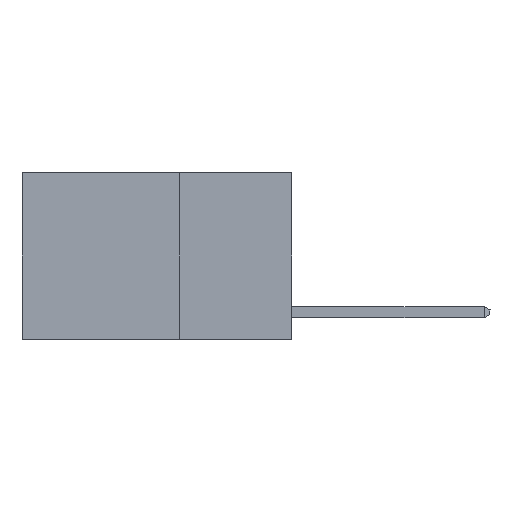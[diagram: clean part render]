
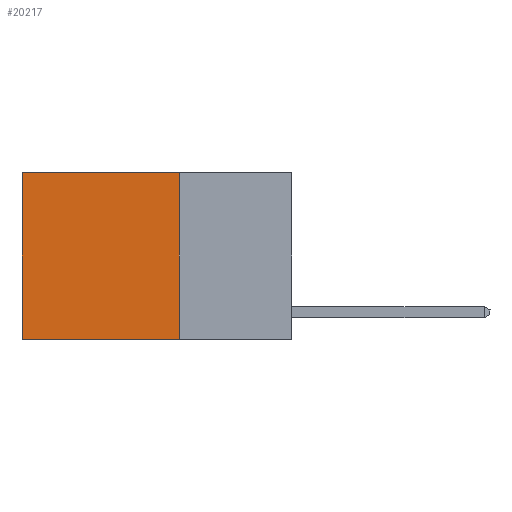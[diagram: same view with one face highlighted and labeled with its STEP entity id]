
A CAD part, left-side view. The second image highlights one B-rep face of the part: STEP entity #20217.
In plain terms, the highlighted planar face has unit normal (-1, 0, 0).
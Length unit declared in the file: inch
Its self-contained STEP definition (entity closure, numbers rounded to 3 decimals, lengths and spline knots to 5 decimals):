
#1565 = LINE ( 'NONE', #19587, #16609 ) ;
#2094 = EDGE_CURVE ( 'NONE', #19064, #14721, #7739, .T. ) ;
#2922 = DIRECTION ( 'NONE',  ( 0., 0., -1. ) ) ;
#3456 = ORIENTED_EDGE ( 'NONE', *, *, #14355, .F. ) ;
#3457 = VECTOR ( 'NONE', #25841, 39.37008 ) ;
#3845 = CARTESIAN_POINT ( 'NONE',  ( 0.2625, 0.25, 0. ) ) ;
#5170 = PLANE ( 'NONE',  #15624 ) ;
#5216 = LINE ( 'NONE', #18605, #3457 ) ;
#5228 = CARTESIAN_POINT ( 'NONE',  ( 0.2625, 0.25, -0.37 ) ) ;
#7739 = LINE ( 'NONE', #5228, #15809 ) ;
#8571 = ORIENTED_EDGE ( 'NONE', *, *, #2094, .F. ) ;
#9744 = CARTESIAN_POINT ( 'NONE',  ( 0.2625, 0.6, 0. ) ) ;
#10278 = VERTEX_POINT ( 'NONE', #9744 ) ;
#10660 = DIRECTION ( 'NONE',  ( 0., 1., 0. ) ) ;
#11819 = ORIENTED_EDGE ( 'NONE', *, *, #25113, .T. ) ;
#12902 = DIRECTION ( 'NONE',  ( 0., 0., -1. ) ) ;
#13089 = CARTESIAN_POINT ( 'NONE',  ( 0.2625, 0.25, 0. ) ) ;
#14293 = DIRECTION ( 'NONE',  ( 0., 1., 0. ) ) ;
#14355 = EDGE_CURVE ( 'NONE', #26585, #19064, #24193, .T. ) ;
#14721 = VERTEX_POINT ( 'NONE', #15954 ) ;
#15624 = AXIS2_PLACEMENT_3D ( 'NONE', #23285, #18989, #2922 ) ;
#15809 = VECTOR ( 'NONE', #14293, 39.37008 ) ;
#15908 = VECTOR ( 'NONE', #12902, 39.37008 ) ;
#15954 = CARTESIAN_POINT ( 'NONE',  ( 0.2625, 0.6, -0.37 ) ) ;
#16609 = VECTOR ( 'NONE', #10660, 39.37008 ) ;
#18605 = CARTESIAN_POINT ( 'NONE',  ( 0.2625, 0.6, 0. ) ) ;
#18989 = DIRECTION ( 'NONE',  ( 1., 0., 0. ) ) ;
#19064 = VERTEX_POINT ( 'NONE', #19579 ) ;
#19579 = CARTESIAN_POINT ( 'NONE',  ( 0.2625, 0.25, -0.37 ) ) ;
#19587 = CARTESIAN_POINT ( 'NONE',  ( 0.2625, 0.25, 0. ) ) ;
#20217 = ADVANCED_FACE ( 'NONE', ( #25650 ), #5170, .F. ) ;
#21531 = ORIENTED_EDGE ( 'NONE', *, *, #22620, .T. ) ;
#22348 = EDGE_LOOP ( 'NONE', ( #11819, #8571, #3456, #21531 ) ) ;
#22620 = EDGE_CURVE ( 'NONE', #26585, #10278, #1565, .T. ) ;
#23285 = CARTESIAN_POINT ( 'NONE',  ( 0.2625, 0.25, 0. ) ) ;
#24193 = LINE ( 'NONE', #3845, #15908 ) ;
#25113 = EDGE_CURVE ( 'NONE', #10278, #14721, #5216, .T. ) ;
#25650 = FACE_OUTER_BOUND ( 'NONE', #22348, .T. ) ;
#25841 = DIRECTION ( 'NONE',  ( 0., 0., -1. ) ) ;
#26585 = VERTEX_POINT ( 'NONE', #13089 ) ;
